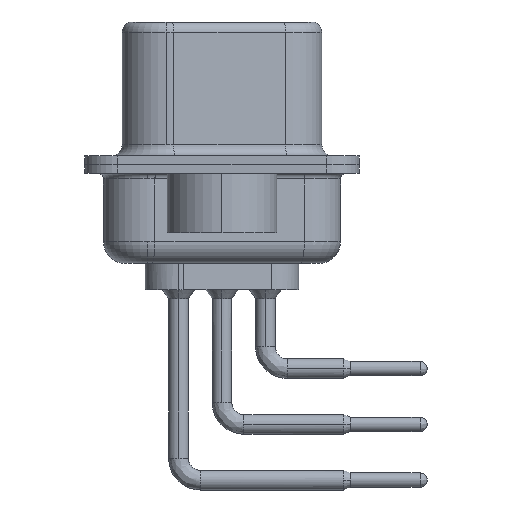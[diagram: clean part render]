
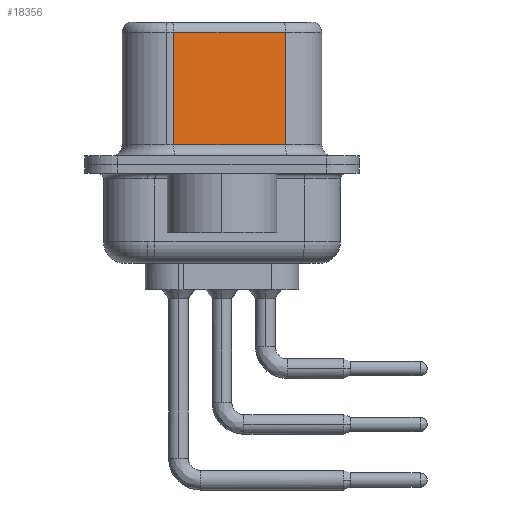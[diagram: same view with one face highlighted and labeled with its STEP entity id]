
A CAD part, left-side view. The second image highlights one B-rep face of the part: STEP entity #18356.
In plain terms, the highlighted planar face has unit normal (-0.985, -0.174, 0).
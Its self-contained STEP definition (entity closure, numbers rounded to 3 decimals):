
#29 = VECTOR ( 'NONE', #5873, 1000. ) ;
#447 = VECTOR ( 'NONE', #15639, 1000. ) ;
#1189 = LINE ( 'NONE', #15599, #447 ) ;
#1618 = CARTESIAN_POINT ( 'NONE',  ( 3.655, 2.203, 0.9 ) ) ;
#2144 = CARTESIAN_POINT ( 'NONE',  ( 3.655, 2.203, 6.02 ) ) ;
#2677 = VECTOR ( 'NONE', #14638, 1000. ) ;
#3615 = AXIS2_PLACEMENT_3D ( 'NONE', #27055, #22798, #9738 ) ;
#4544 = CARTESIAN_POINT ( 'NONE',  ( 4.555, -2.897, 0.9 ) ) ;
#5873 = DIRECTION ( 'NONE',  ( 0., 0., -1. ) ) ;
#6100 = LINE ( 'NONE', #27585, #29 ) ;
#6317 = EDGE_CURVE ( 'NONE', #14189, #16133, #1189, .T. ) ;
#6593 = ORIENTED_EDGE ( 'NONE', *, *, #13318, .T. ) ;
#7534 = PLANE ( 'NONE',  #3615 ) ;
#7923 = DIRECTION ( 'NONE',  ( 0.174, -0.985, 0. ) ) ;
#8306 = VECTOR ( 'NONE', #7923, 1000. ) ;
#8353 = ORIENTED_EDGE ( 'NONE', *, *, #6317, .T. ) ;
#8567 = LINE ( 'NONE', #27708, #2677 ) ;
#9378 = CARTESIAN_POINT ( 'NONE',  ( 4.555, -2.897, 6.02 ) ) ;
#9738 = DIRECTION ( 'NONE',  ( -0.174, 0.985, 0. ) ) ;
#11617 = FACE_OUTER_BOUND ( 'NONE', #22587, .T. ) ;
#11764 = EDGE_CURVE ( 'NONE', #24809, #23780, #25694, .T. ) ;
#13318 = EDGE_CURVE ( 'NONE', #16133, #24809, #8567, .T. ) ;
#14189 = VERTEX_POINT ( 'NONE', #9378 ) ;
#14638 = DIRECTION ( 'NONE',  ( 0., 0., -1. ) ) ;
#15599 = CARTESIAN_POINT ( 'NONE',  ( 4.555, -2.897, 6.02 ) ) ;
#15639 = DIRECTION ( 'NONE',  ( -0.174, 0.985, 0. ) ) ;
#16133 = VERTEX_POINT ( 'NONE', #2144 ) ;
#16570 = CARTESIAN_POINT ( 'NONE',  ( 4.555, -2.897, 0.9 ) ) ;
#18356 = ADVANCED_FACE ( 'NONE', ( #11617 ), #7534, .F. ) ;
#18849 = ORIENTED_EDGE ( 'NONE', *, *, #11764, .T. ) ;
#19092 = EDGE_CURVE ( 'NONE', #14189, #23780, #6100, .T. ) ;
#21772 = ORIENTED_EDGE ( 'NONE', *, *, #19092, .F. ) ;
#22587 = EDGE_LOOP ( 'NONE', ( #21772, #8353, #6593, #18849 ) ) ;
#22798 = DIRECTION ( 'NONE',  ( 0.985, 0.174, 0. ) ) ;
#23780 = VERTEX_POINT ( 'NONE', #4544 ) ;
#24809 = VERTEX_POINT ( 'NONE', #1618 ) ;
#25694 = LINE ( 'NONE', #16570, #8306 ) ;
#27055 = CARTESIAN_POINT ( 'NONE',  ( 4.555, -2.897, 6.52 ) ) ;
#27585 = CARTESIAN_POINT ( 'NONE',  ( 4.555, -2.897, 6.52 ) ) ;
#27708 = CARTESIAN_POINT ( 'NONE',  ( 3.655, 2.203, 6.52 ) ) ;
